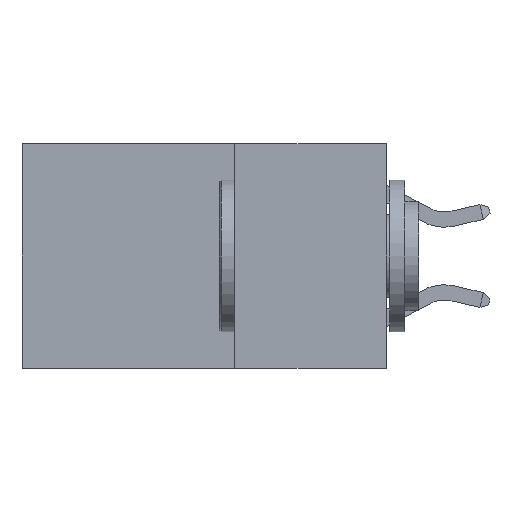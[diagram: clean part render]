
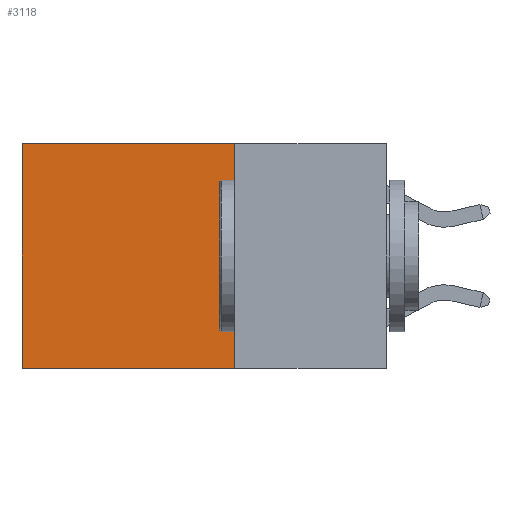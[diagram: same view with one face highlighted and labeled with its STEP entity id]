
A CAD part, left-side view. The second image highlights one B-rep face of the part: STEP entity #3118.
In plain terms, the highlighted planar face has unit normal (-1, 0, 0).
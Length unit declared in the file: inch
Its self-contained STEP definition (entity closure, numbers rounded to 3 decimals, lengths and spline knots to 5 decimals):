
#849 = CARTESIAN_POINT ( 'NONE',  ( 0.2625, 0.6, 0. ) ) ;
#1291 = LINE ( 'NONE', #7679, #8828 ) ;
#1469 = CARTESIAN_POINT ( 'NONE',  ( 0.2625, 0.25, 0. ) ) ;
#2029 = VECTOR ( 'NONE', #9236, 39.37008 ) ;
#2049 = ORIENTED_EDGE ( 'NONE', *, *, #5799, .F. ) ;
#2279 = DIRECTION ( 'NONE',  ( 0., 1., 0. ) ) ;
#2434 = DIRECTION ( 'NONE',  ( 0., 0., -1. ) ) ;
#2708 = CARTESIAN_POINT ( 'NONE',  ( 0.2625, 0.25, -0.37 ) ) ;
#2728 = EDGE_CURVE ( 'NONE', #7100, #9777, #2836, .T. ) ;
#2836 = LINE ( 'NONE', #3870, #6600 ) ;
#3118 = ADVANCED_FACE ( 'NONE', ( #9895 ), #9136, .F. ) ;
#3482 = CARTESIAN_POINT ( 'NONE',  ( 0.2625, 0.25, 0. ) ) ;
#3870 = CARTESIAN_POINT ( 'NONE',  ( 0.2625, 0.6, 0. ) ) ;
#4166 = ORIENTED_EDGE ( 'NONE', *, *, #2728, .T. ) ;
#4213 = AXIS2_PLACEMENT_3D ( 'NONE', #1469, #7015, #2434 ) ;
#4368 = LINE ( 'NONE', #3482, #2029 ) ;
#4872 = EDGE_CURVE ( 'NONE', #7071, #9777, #1291, .T. ) ;
#5022 = CARTESIAN_POINT ( 'NONE',  ( 0.2625, 0.6, -0.37 ) ) ;
#5619 = LINE ( 'NONE', #8847, #9215 ) ;
#5799 = EDGE_CURVE ( 'NONE', #5966, #7071, #4368, .T. ) ;
#5966 = VERTEX_POINT ( 'NONE', #8610 ) ;
#6230 = ORIENTED_EDGE ( 'NONE', *, *, #8621, .T. ) ;
#6387 = EDGE_LOOP ( 'NONE', ( #4166, #9796, #2049, #6230 ) ) ;
#6600 = VECTOR ( 'NONE', #9554, 39.37008 ) ;
#6712 = DIRECTION ( 'NONE',  ( 0., 1., 0. ) ) ;
#7015 = DIRECTION ( 'NONE',  ( 1., 0., 0. ) ) ;
#7071 = VERTEX_POINT ( 'NONE', #2708 ) ;
#7100 = VERTEX_POINT ( 'NONE', #849 ) ;
#7679 = CARTESIAN_POINT ( 'NONE',  ( 0.2625, 0.25, -0.37 ) ) ;
#8610 = CARTESIAN_POINT ( 'NONE',  ( 0.2625, 0.25, 0. ) ) ;
#8621 = EDGE_CURVE ( 'NONE', #5966, #7100, #5619, .T. ) ;
#8828 = VECTOR ( 'NONE', #2279, 39.37008 ) ;
#8847 = CARTESIAN_POINT ( 'NONE',  ( 0.2625, 0.25, 0. ) ) ;
#9136 = PLANE ( 'NONE',  #4213 ) ;
#9215 = VECTOR ( 'NONE', #6712, 39.37008 ) ;
#9236 = DIRECTION ( 'NONE',  ( 0., 0., -1. ) ) ;
#9554 = DIRECTION ( 'NONE',  ( 0., 0., -1. ) ) ;
#9777 = VERTEX_POINT ( 'NONE', #5022 ) ;
#9796 = ORIENTED_EDGE ( 'NONE', *, *, #4872, .F. ) ;
#9895 = FACE_OUTER_BOUND ( 'NONE', #6387, .T. ) ;
